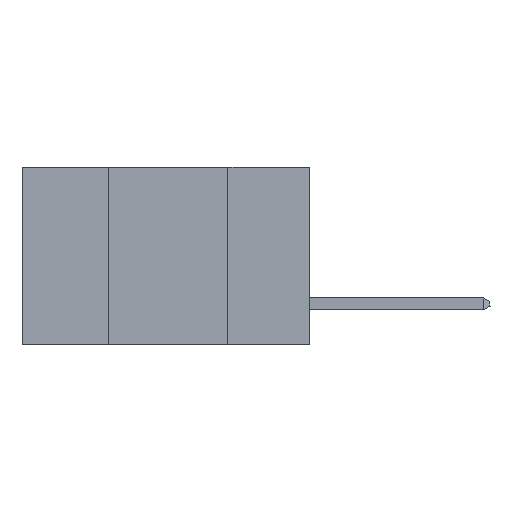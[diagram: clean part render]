
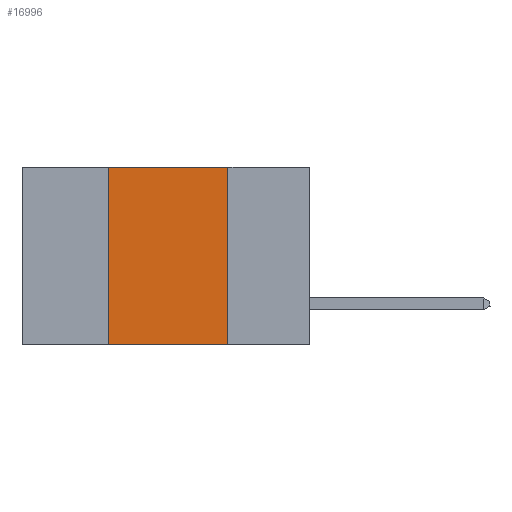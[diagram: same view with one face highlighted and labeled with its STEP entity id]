
A CAD part, left-side view. The second image highlights one B-rep face of the part: STEP entity #16996.
In plain terms, the highlighted planar face has unit normal (-1, 0, 0).
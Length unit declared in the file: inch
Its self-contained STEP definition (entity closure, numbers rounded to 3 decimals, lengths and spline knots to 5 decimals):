
#1575 = CARTESIAN_POINT ( 'NONE',  ( 0., 0.6, -0.37 ) ) ;
#2783 = DIRECTION ( 'NONE',  ( 0., -1., 0. ) ) ;
#2980 = AXIS2_PLACEMENT_3D ( 'NONE', #4927, #44384, #11555 ) ;
#3067 = CARTESIAN_POINT ( 'NONE',  ( 0., 0.17, -0.37 ) ) ;
#4927 = CARTESIAN_POINT ( 'NONE',  ( 0., 0.6, 0. ) ) ;
#6029 = DIRECTION ( 'NONE',  ( 0., 0., 1. ) ) ;
#8284 = EDGE_LOOP ( 'NONE', ( #39244, #15827, #9538, #36602 ) ) ;
#9538 = ORIENTED_EDGE ( 'NONE', *, *, #21043, .F. ) ;
#9980 = VECTOR ( 'NONE', #41579, 39.37008 ) ;
#10086 = FACE_OUTER_BOUND ( 'NONE', #8284, .T. ) ;
#11068 = LINE ( 'NONE', #45083, #9980 ) ;
#11555 = DIRECTION ( 'NONE',  ( 0., 0., -1. ) ) ;
#14579 = CARTESIAN_POINT ( 'NONE',  ( 0., 0.42, 0. ) ) ;
#15827 = ORIENTED_EDGE ( 'NONE', *, *, #45850, .F. ) ;
#16706 = VECTOR ( 'NONE', #6029, 39.37008 ) ;
#16996 = ADVANCED_FACE ( 'NONE', ( #10086 ), #39806, .F. ) ;
#21043 = EDGE_CURVE ( 'NONE', #22865, #36439, #26265, .T. ) ;
#22865 = VERTEX_POINT ( 'NONE', #23321 ) ;
#23321 = CARTESIAN_POINT ( 'NONE',  ( 0., 0.42, -0.37 ) ) ;
#26265 = LINE ( 'NONE', #41640, #16706 ) ;
#27960 = VECTOR ( 'NONE', #2783, 39.37008 ) ;
#29142 = EDGE_CURVE ( 'NONE', #29248, #39351, #11068, .T. ) ;
#29248 = VERTEX_POINT ( 'NONE', #46071 ) ;
#30673 = LINE ( 'NONE', #1575, #39055 ) ;
#30774 = EDGE_CURVE ( 'NONE', #22865, #39351, #30673, .T. ) ;
#33964 = DIRECTION ( 'NONE',  ( 0., -1., 0. ) ) ;
#36439 = VERTEX_POINT ( 'NONE', #14579 ) ;
#36602 = ORIENTED_EDGE ( 'NONE', *, *, #30774, .T. ) ;
#37577 = CARTESIAN_POINT ( 'NONE',  ( 0., 0.6, 0. ) ) ;
#39055 = VECTOR ( 'NONE', #33964, 39.37008 ) ;
#39244 = ORIENTED_EDGE ( 'NONE', *, *, #29142, .F. ) ;
#39351 = VERTEX_POINT ( 'NONE', #3067 ) ;
#39806 = PLANE ( 'NONE',  #2980 ) ;
#41579 = DIRECTION ( 'NONE',  ( 0., 0., -1. ) ) ;
#41640 = CARTESIAN_POINT ( 'NONE',  ( 0., 0.42, 0. ) ) ;
#43630 = LINE ( 'NONE', #37577, #27960 ) ;
#44384 = DIRECTION ( 'NONE',  ( 1., 0., 0. ) ) ;
#45083 = CARTESIAN_POINT ( 'NONE',  ( 0., 0.17, 0. ) ) ;
#45850 = EDGE_CURVE ( 'NONE', #36439, #29248, #43630, .T. ) ;
#46071 = CARTESIAN_POINT ( 'NONE',  ( 0., 0.17, 0. ) ) ;
